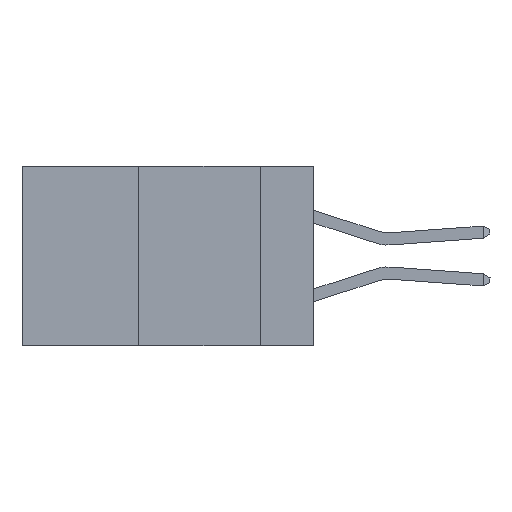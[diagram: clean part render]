
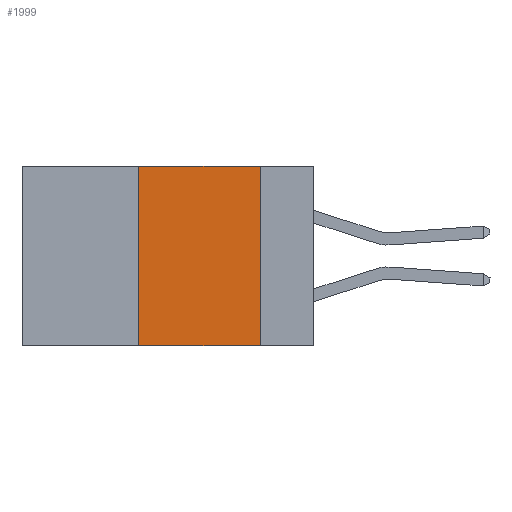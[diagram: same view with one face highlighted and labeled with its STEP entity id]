
A CAD part, left-side view. The second image highlights one B-rep face of the part: STEP entity #1999.
In plain terms, the highlighted planar face has unit normal (-1, 0, 0).
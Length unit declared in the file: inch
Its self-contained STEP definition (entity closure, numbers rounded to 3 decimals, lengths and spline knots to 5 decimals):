
#229 = VERTEX_POINT ( 'NONE', #3524 ) ;
#565 = ORIENTED_EDGE ( 'NONE', *, *, #6459, .F. ) ;
#943 = EDGE_CURVE ( 'NONE', #1170, #7838, #9853, .T. ) ;
#1170 = VERTEX_POINT ( 'NONE', #1411 ) ;
#1262 = CARTESIAN_POINT ( 'NONE',  ( 0., 0.36, 0. ) ) ;
#1411 = CARTESIAN_POINT ( 'NONE',  ( 0., 0.11, 0. ) ) ;
#1498 = AXIS2_PLACEMENT_3D ( 'NONE', #7920, #3252, #3558 ) ;
#1999 = ADVANCED_FACE ( 'NONE', ( #4055 ), #10252, .F. ) ;
#2266 = DIRECTION ( 'NONE',  ( 0., 0., 1. ) ) ;
#2551 = EDGE_CURVE ( 'NONE', #4279, #229, #7293, .T. ) ;
#3252 = DIRECTION ( 'NONE',  ( 1., 0., 0. ) ) ;
#3524 = CARTESIAN_POINT ( 'NONE',  ( 0., 0.36, 0. ) ) ;
#3558 = DIRECTION ( 'NONE',  ( 0., 0., -1. ) ) ;
#3959 = LINE ( 'NONE', #11040, #8234 ) ;
#4055 = FACE_OUTER_BOUND ( 'NONE', #5024, .T. ) ;
#4279 = VERTEX_POINT ( 'NONE', #9512 ) ;
#4370 = ORIENTED_EDGE ( 'NONE', *, *, #6005, .T. ) ;
#5024 = EDGE_LOOP ( 'NONE', ( #5508, #565, #8688, #4370 ) ) ;
#5508 = ORIENTED_EDGE ( 'NONE', *, *, #943, .F. ) ;
#5599 = CARTESIAN_POINT ( 'NONE',  ( 0., 0.6, 0. ) ) ;
#5889 = CARTESIAN_POINT ( 'NONE',  ( 0., 0.11, -0.37 ) ) ;
#6005 = EDGE_CURVE ( 'NONE', #4279, #7838, #3959, .T. ) ;
#6459 = EDGE_CURVE ( 'NONE', #229, #1170, #10622, .T. ) ;
#6548 = VECTOR ( 'NONE', #8153, 39.37008 ) ;
#6942 = DIRECTION ( 'NONE',  ( 0., -1., 0. ) ) ;
#7293 = LINE ( 'NONE', #1262, #9194 ) ;
#7838 = VERTEX_POINT ( 'NONE', #5889 ) ;
#7920 = CARTESIAN_POINT ( 'NONE',  ( 0., 0.6, 0. ) ) ;
#8153 = DIRECTION ( 'NONE',  ( 0., -1., 0. ) ) ;
#8234 = VECTOR ( 'NONE', #6942, 39.37008 ) ;
#8688 = ORIENTED_EDGE ( 'NONE', *, *, #2551, .F. ) ;
#9194 = VECTOR ( 'NONE', #2266, 39.37008 ) ;
#9279 = CARTESIAN_POINT ( 'NONE',  ( 0., 0.11, 0. ) ) ;
#9512 = CARTESIAN_POINT ( 'NONE',  ( 0., 0.36, -0.37 ) ) ;
#9853 = LINE ( 'NONE', #9279, #10605 ) ;
#10144 = DIRECTION ( 'NONE',  ( 0., 0., -1. ) ) ;
#10252 = PLANE ( 'NONE',  #1498 ) ;
#10605 = VECTOR ( 'NONE', #10144, 39.37008 ) ;
#10622 = LINE ( 'NONE', #5599, #6548 ) ;
#11040 = CARTESIAN_POINT ( 'NONE',  ( 0., 0.6, -0.37 ) ) ;
